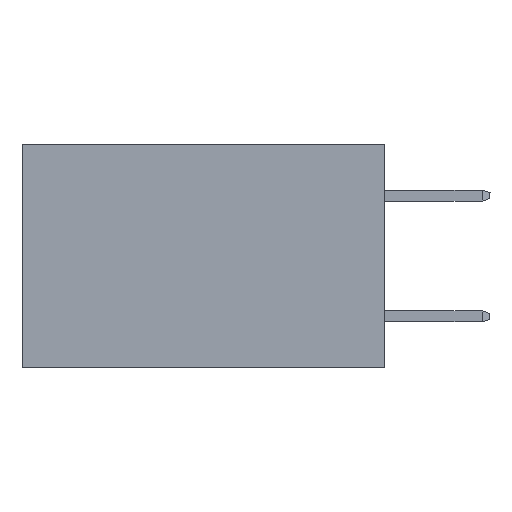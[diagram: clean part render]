
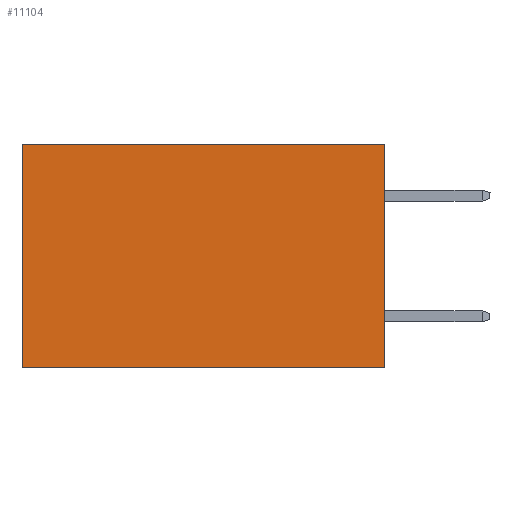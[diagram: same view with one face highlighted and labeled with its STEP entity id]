
A CAD part, left-side view. The second image highlights one B-rep face of the part: STEP entity #11104.
In plain terms, the highlighted planar face has unit normal (-1, 0, 0).
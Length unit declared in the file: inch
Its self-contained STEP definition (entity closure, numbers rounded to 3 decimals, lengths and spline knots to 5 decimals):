
#94 = EDGE_CURVE ( 'NONE', #11550, #11544, #8070, .T. ) ;
#505 = CARTESIAN_POINT ( 'NONE',  ( 0.298, 0., 0. ) ) ;
#530 = ORIENTED_EDGE ( 'NONE', *, *, #94, .F. ) ;
#594 = ORIENTED_EDGE ( 'NONE', *, *, #6349, .F. ) ;
#956 = VECTOR ( 'NONE', #7554, 39.37008 ) ;
#1223 = DIRECTION ( 'NONE',  ( 0., 0., -1. ) ) ;
#2341 = DIRECTION ( 'NONE',  ( 0., 1., 0. ) ) ;
#2834 = VECTOR ( 'NONE', #2341, 39.37008 ) ;
#3461 = CARTESIAN_POINT ( 'NONE',  ( 0.298, 0.6, -0.37 ) ) ;
#3664 = ORIENTED_EDGE ( 'NONE', *, *, #11318, .T. ) ;
#4387 = CARTESIAN_POINT ( 'NONE',  ( 0.298, 0., -0.37 ) ) ;
#4686 = PLANE ( 'NONE',  #11920 ) ;
#5905 = LINE ( 'NONE', #8426, #956 ) ;
#5998 = DIRECTION ( 'NONE',  ( 0., 1., 0. ) ) ;
#6140 = VECTOR ( 'NONE', #1223, 39.37008 ) ;
#6220 = VERTEX_POINT ( 'NONE', #11515 ) ;
#6349 = EDGE_CURVE ( 'NONE', #11544, #11680, #8086, .T. ) ;
#6500 = CARTESIAN_POINT ( 'NONE',  ( 0.298, 0., 0. ) ) ;
#7362 = CARTESIAN_POINT ( 'NONE',  ( 0.298, 0., 0. ) ) ;
#7554 = DIRECTION ( 'NONE',  ( 0., 0., -1. ) ) ;
#7927 = EDGE_LOOP ( 'NONE', ( #9375, #594, #530, #3664 ) ) ;
#8070 = LINE ( 'NONE', #10392, #6140 ) ;
#8086 = LINE ( 'NONE', #8700, #8973 ) ;
#8426 = CARTESIAN_POINT ( 'NONE',  ( 0.298, 0.6, 0. ) ) ;
#8700 = CARTESIAN_POINT ( 'NONE',  ( 0.298, 0., -0.37 ) ) ;
#8973 = VECTOR ( 'NONE', #5998, 39.37008 ) ;
#9349 = DIRECTION ( 'NONE',  ( 1., 0., 0. ) ) ;
#9375 = ORIENTED_EDGE ( 'NONE', *, *, #10319, .T. ) ;
#10319 = EDGE_CURVE ( 'NONE', #6220, #11680, #5905, .T. ) ;
#10392 = CARTESIAN_POINT ( 'NONE',  ( 0.298, 0., 0. ) ) ;
#10449 = LINE ( 'NONE', #505, #2834 ) ;
#11104 = ADVANCED_FACE ( 'NONE', ( #11324 ), #4686, .F. ) ;
#11234 = DIRECTION ( 'NONE',  ( 0., 0., -1. ) ) ;
#11318 = EDGE_CURVE ( 'NONE', #11550, #6220, #10449, .T. ) ;
#11324 = FACE_OUTER_BOUND ( 'NONE', #7927, .T. ) ;
#11515 = CARTESIAN_POINT ( 'NONE',  ( 0.298, 0.6, 0. ) ) ;
#11544 = VERTEX_POINT ( 'NONE', #4387 ) ;
#11550 = VERTEX_POINT ( 'NONE', #7362 ) ;
#11680 = VERTEX_POINT ( 'NONE', #3461 ) ;
#11920 = AXIS2_PLACEMENT_3D ( 'NONE', #6500, #9349, #11234 ) ;
